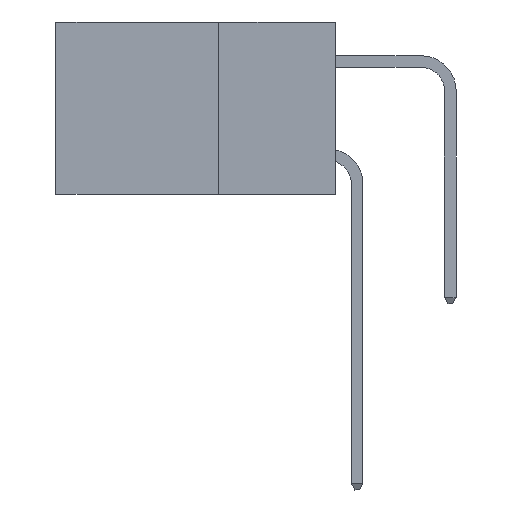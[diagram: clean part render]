
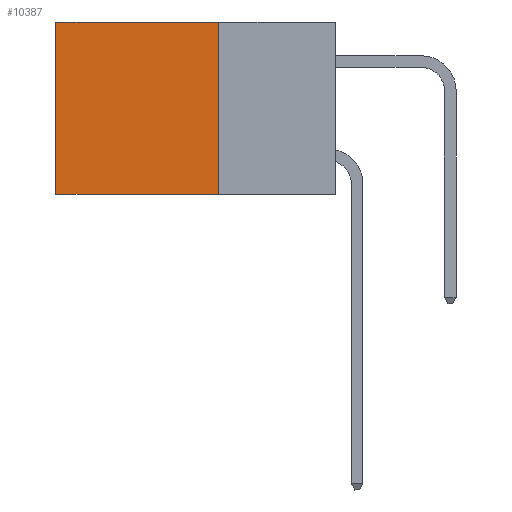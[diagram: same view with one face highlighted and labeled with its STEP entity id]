
A CAD part, left-side view. The second image highlights one B-rep face of the part: STEP entity #10387.
In plain terms, the highlighted planar face has unit normal (-1, 0, 0).
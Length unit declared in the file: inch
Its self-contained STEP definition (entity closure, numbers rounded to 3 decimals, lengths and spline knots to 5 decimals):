
#139 = CARTESIAN_POINT ( 'NONE',  ( 0.2875, 0.25, -0.37 ) ) ;
#272 = LINE ( 'NONE', #1154, #6087 ) ;
#358 = CARTESIAN_POINT ( 'NONE',  ( 0.2875, 0.25, 0. ) ) ;
#426 = VECTOR ( 'NONE', #11416, 39.37008 ) ;
#655 = EDGE_CURVE ( 'NONE', #5800, #9565, #9426, .T. ) ;
#656 = EDGE_LOOP ( 'NONE', ( #10353, #3007, #3358, #7601 ) ) ;
#841 = EDGE_CURVE ( 'NONE', #8838, #12025, #1933, .T. ) ;
#941 = DIRECTION ( 'NONE',  ( 0., 0., -1. ) ) ;
#1154 = CARTESIAN_POINT ( 'NONE',  ( 0.2875, 0.6, 0. ) ) ;
#1593 = VECTOR ( 'NONE', #9828, 39.37008 ) ;
#1933 = LINE ( 'NONE', #139, #426 ) ;
#2924 = CARTESIAN_POINT ( 'NONE',  ( 0.2875, 0.25, 0. ) ) ;
#3007 = ORIENTED_EDGE ( 'NONE', *, *, #841, .F. ) ;
#3358 = ORIENTED_EDGE ( 'NONE', *, *, #5911, .F. ) ;
#4071 = CARTESIAN_POINT ( 'NONE',  ( 0.2875, 0.25, 0. ) ) ;
#4211 = CARTESIAN_POINT ( 'NONE',  ( 0.2875, 0.6, -0.37 ) ) ;
#4943 = EDGE_CURVE ( 'NONE', #9565, #12025, #272, .T. ) ;
#5244 = LINE ( 'NONE', #358, #1593 ) ;
#5800 = VERTEX_POINT ( 'NONE', #4071 ) ;
#5911 = EDGE_CURVE ( 'NONE', #5800, #8838, #5244, .T. ) ;
#6087 = VECTOR ( 'NONE', #8614, 39.37008 ) ;
#6632 = CARTESIAN_POINT ( 'NONE',  ( 0.2875, 0.25, 0. ) ) ;
#7586 = CARTESIAN_POINT ( 'NONE',  ( 0.2875, 0.6, 0. ) ) ;
#7601 = ORIENTED_EDGE ( 'NONE', *, *, #655, .T. ) ;
#7745 = PLANE ( 'NONE',  #9589 ) ;
#7926 = VECTOR ( 'NONE', #10487, 39.37008 ) ;
#8614 = DIRECTION ( 'NONE',  ( 0., 0., -1. ) ) ;
#8838 = VERTEX_POINT ( 'NONE', #9839 ) ;
#9426 = LINE ( 'NONE', #2924, #7926 ) ;
#9565 = VERTEX_POINT ( 'NONE', #7586 ) ;
#9589 = AXIS2_PLACEMENT_3D ( 'NONE', #6632, #11550, #941 ) ;
#9828 = DIRECTION ( 'NONE',  ( 0., 0., -1. ) ) ;
#9839 = CARTESIAN_POINT ( 'NONE',  ( 0.2875, 0.25, -0.37 ) ) ;
#10353 = ORIENTED_EDGE ( 'NONE', *, *, #4943, .T. ) ;
#10387 = ADVANCED_FACE ( 'NONE', ( #11412 ), #7745, .F. ) ;
#10487 = DIRECTION ( 'NONE',  ( 0., 1., 0. ) ) ;
#11412 = FACE_OUTER_BOUND ( 'NONE', #656, .T. ) ;
#11416 = DIRECTION ( 'NONE',  ( 0., 1., 0. ) ) ;
#11550 = DIRECTION ( 'NONE',  ( 1., 0., 0. ) ) ;
#12025 = VERTEX_POINT ( 'NONE', #4211 ) ;
